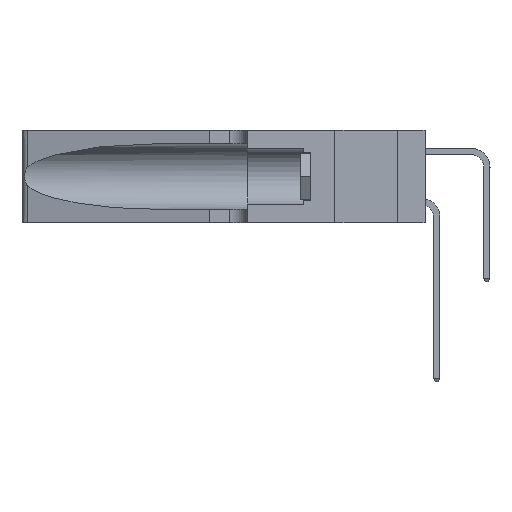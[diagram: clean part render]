
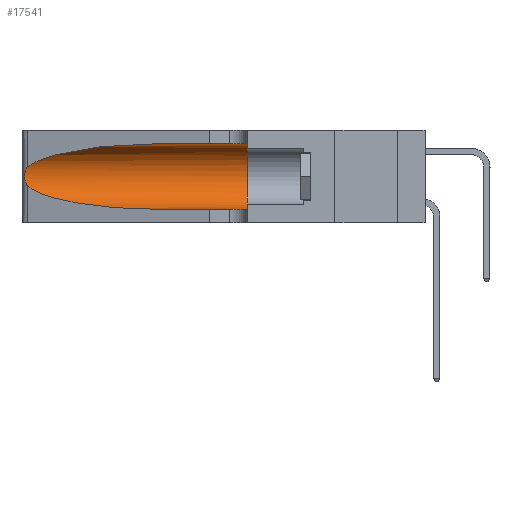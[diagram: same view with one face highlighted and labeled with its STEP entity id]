
A CAD part, left-side view. The second image highlights one B-rep face of the part: STEP entity #17541.
In plain terms, the highlighted cylindrical face has radius 3.308 mm (diameter 6.617 mm), a partial arc.
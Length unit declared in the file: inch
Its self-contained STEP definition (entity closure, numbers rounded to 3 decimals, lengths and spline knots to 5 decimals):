
#301 = CARTESIAN_POINT ( 'NONE',  ( 0.25854, 1.2359, 0.20912 ) ) ;
#621 = CARTESIAN_POINT ( 'NONE',  ( 0.25487, 1.22718, 0.22369 ) ) ;
#2747 = LINE ( 'NONE', #35736, #3818 ) ;
#3152 = EDGE_CURVE ( 'NONE', #33788, #25745, #2747, .T. ) ;
#3167 = FACE_OUTER_BOUND ( 'NONE', #29818, .T. ) ;
#3712 = CARTESIAN_POINT ( 'NONE',  ( 0.26075, 1.23896, 0.19203 ) ) ;
#3818 = VECTOR ( 'NONE', #15447, 39.37008 ) ;
#5993 = CARTESIAN_POINT ( 'NONE',  ( 0.1305, 0.72297, 0.05475 ) ) ;
#6169 = CARTESIAN_POINT ( 'NONE',  ( 0.1305, 0.35, 0.31525 ) ) ;
#7078 = ORIENTED_EDGE ( 'NONE', *, *, #19544, .T. ) ;
#7153 = CARTESIAN_POINT ( 'NONE',  ( 0.26017, 1.23833, 0.17102 ) ) ;
#7321 = CARTESIAN_POINT ( 'NONE',  ( 0.1305, 0.72297, 0.31525 ) ) ;
#7990 = VERTEX_POINT ( 'NONE', #5993 ) ;
#8357 = DIRECTION ( 'NONE',  ( 0., -1., 0. ) ) ;
#9661 = VECTOR ( 'NONE', #30434, 39.37008 ) ;
#10611 = CARTESIAN_POINT ( 'NONE',  ( 0.25789, 1.23486, 0.15765 ) ) ;
#12735 = CARTESIAN_POINT ( 'NONE',  ( 0.25487, 1.22718, 0.14631 ) ) ;
#12739 = CARTESIAN_POINT ( 'NONE',  ( 0.2373, 1.15595, 0.08982 ) ) ;
#13386 = CARTESIAN_POINT ( 'NONE',  ( 0.1305, 1.61858, 0.05475 ) ) ;
#14076 = CARTESIAN_POINT ( 'NONE',  ( 0.25555, 1.22993, 0.14849 ) ) ;
#15447 = DIRECTION ( 'NONE',  ( 0., -1., 0. ) ) ;
#15853 = ORIENTED_EDGE ( 'NONE', *, *, #41350, .T. ) ;
#16373 = EDGE_CURVE ( 'NONE', #31838, #41891, #40515, .T. ) ;
#17353 = CARTESIAN_POINT ( 'NONE',  ( 0.25487, 1.22718, 0.22369 ) ) ;
#17355 = CARTESIAN_POINT ( 'NONE',  ( 0.1305, 0.35, 0.185 ) ) ;
#17541 = ADVANCED_FACE ( 'NONE', ( #3167 ), #20293, .F. ) ;
#19483 = CIRCLE ( 'NONE', #40063, 0.13025 ) ;
#19544 = EDGE_CURVE ( 'NONE', #41891, #7990, #32634, .T. ) ;
#19593 = CARTESIAN_POINT ( 'NONE',  ( 0.18966, 0.96281, 0.05475 ) ) ;
#20293 = CYLINDRICAL_SURFACE ( 'NONE', #39817, 0.13025 ) ;
#20771 = CARTESIAN_POINT ( 'NONE',  ( 0.25787, 1.23484, 0.2124 ) ) ;
#20772 = DIRECTION ( 'NONE',  ( 0., 0., 1. ) ) ;
#21089 = CARTESIAN_POINT ( 'NONE',  ( 0.2373, 1.15595, 0.28018 ) ) ;
#21421 = ORIENTED_EDGE ( 'NONE', *, *, #38434, .T. ) ;
#23012 = CARTESIAN_POINT ( 'NONE',  ( 0.1305, 0.72297, 0.31525 ) ) ;
#24134 = CARTESIAN_POINT ( 'NONE',  ( 0.26018, 1.23835, 0.19895 ) ) ;
#25485 = CARTESIAN_POINT ( 'NONE',  ( 0.1305, 1.61858, 0.185 ) ) ;
#25745 = VERTEX_POINT ( 'NONE', #6169 ) ;
#26051 = ORIENTED_EDGE ( 'NONE', *, *, #28707, .F. ) ;
#26165 = CARTESIAN_POINT ( 'NONE',  ( 0.25487, 1.22718, 0.22369 ) ) ;
#26669 = LINE ( 'NONE', #13386, #9661 ) ;
#27541 = CARTESIAN_POINT ( 'NONE',  ( 0.26075, 1.23896, 0.178 ) ) ;
#28707 = EDGE_CURVE ( 'NONE', #25745, #42920, #19483, .T. ) ;
#28736 = ORIENTED_EDGE ( 'NONE', *, *, #3152, .F. ) ;
#29818 = EDGE_LOOP ( 'NONE', ( #21421, #42593, #7078, #15853, #26051, #28736 ) ) ;
#30434 = DIRECTION ( 'NONE',  ( 0., -1., 0. ) ) ;
#30961 = CARTESIAN_POINT ( 'NONE',  ( 0.25856, 1.23593, 0.16098 ) ) ;
#31838 = VERTEX_POINT ( 'NONE', #26165 ) ;
#32175 = DIRECTION ( 'NONE',  ( 0., 0., -1. ) ) ;
#32634 =( BOUNDED_CURVE ( )  B_SPLINE_CURVE ( 3, ( #36473, #12739, #19593, #43334 ),
 .UNSPECIFIED., .F., .T. ) 
 B_SPLINE_CURVE_WITH_KNOTS ( ( 4, 4 ),
 ( 3.44316, 4.71239 ),
 .UNSPECIFIED. ) 
 CURVE ( )  GEOMETRIC_REPRESENTATION_ITEM ( )  RATIONAL_B_SPLINE_CURVE ( ( 1., 0.87, 0.87, 1. ) ) 
 REPRESENTATION_ITEM ( '' )  );
#33788 = VERTEX_POINT ( 'NONE', #23012 ) ;
#34383 = CARTESIAN_POINT ( 'NONE',  ( 0.25639, 1.23186, 0.15144 ) ) ;
#35736 = CARTESIAN_POINT ( 'NONE',  ( 0.1305, 1.61858, 0.31525 ) ) ;
#36473 = CARTESIAN_POINT ( 'NONE',  ( 0.25487, 1.22718, 0.14631 ) ) ;
#37624 = CARTESIAN_POINT ( 'NONE',  ( 0.25555, 1.22994, 0.2215 ) ) ;
#37773 = CARTESIAN_POINT ( 'NONE',  ( 0.25487, 1.22718, 0.14631 ) ) ;
#37790 = CARTESIAN_POINT ( 'NONE',  ( 0.1305, 0.35, 0.05475 ) ) ;
#38434 = EDGE_CURVE ( 'NONE', #33788, #31838, #41880, .T. ) ;
#39817 = AXIS2_PLACEMENT_3D ( 'NONE', #25485, #8357, #32175 ) ;
#40063 = AXIS2_PLACEMENT_3D ( 'NONE', #17355, #41063, #20772 ) ;
#40515 = B_SPLINE_CURVE_WITH_KNOTS ( 'NONE', 3,
 ( #17353, #37624, #41060, #20771, #301, #24134, #3712, #27541, #7153, #30961, #10611, #34383, #14076, #37773 ),
 .UNSPECIFIED., .F., .F.,
 ( 4, 2, 2, 2, 2, 2, 4 ),
 ( 0., 0.00027, 0.00053, 0.00107, 0.0016, 0.00187, 0.00214 ),
 .UNSPECIFIED. ) ;
#41060 = CARTESIAN_POINT ( 'NONE',  ( 0.25639, 1.23184, 0.21858 ) ) ;
#41063 = DIRECTION ( 'NONE',  ( 0., 1., 0. ) ) ;
#41350 = EDGE_CURVE ( 'NONE', #7990, #42920, #26669, .T. ) ;
#41390 = CARTESIAN_POINT ( 'NONE',  ( 0.18966, 0.96281, 0.31525 ) ) ;
#41880 =( BOUNDED_CURVE ( )  B_SPLINE_CURVE ( 3, ( #7321, #41390, #21089, #621 ),
 .UNSPECIFIED., .F., .F. ) 
 B_SPLINE_CURVE_WITH_KNOTS ( ( 4, 4 ),
 ( 1.5708, 2.84003 ),
 .UNSPECIFIED. ) 
 CURVE ( )  GEOMETRIC_REPRESENTATION_ITEM ( )  RATIONAL_B_SPLINE_CURVE ( ( 1., 0.87, 0.87, 1. ) ) 
 REPRESENTATION_ITEM ( '' )  );
#41891 = VERTEX_POINT ( 'NONE', #12735 ) ;
#42593 = ORIENTED_EDGE ( 'NONE', *, *, #16373, .T. ) ;
#42920 = VERTEX_POINT ( 'NONE', #37790 ) ;
#43334 = CARTESIAN_POINT ( 'NONE',  ( 0.1305, 0.72297, 0.05475 ) ) ;
